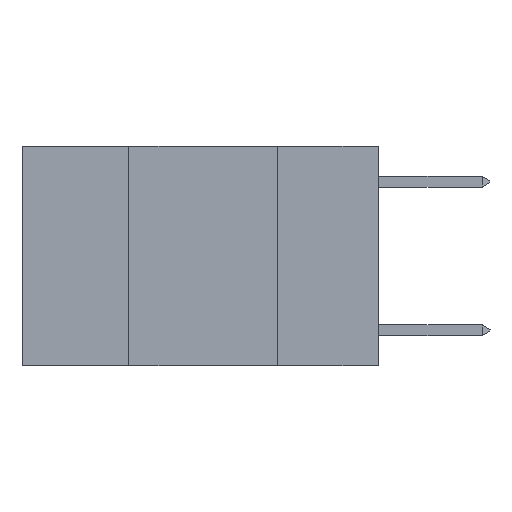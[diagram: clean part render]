
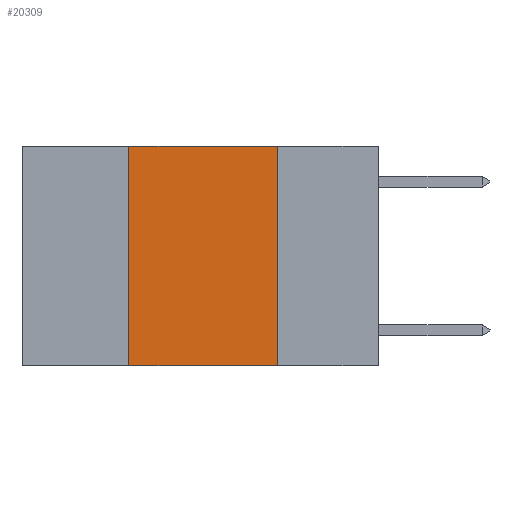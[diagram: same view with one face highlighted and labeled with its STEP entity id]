
A CAD part, left-side view. The second image highlights one B-rep face of the part: STEP entity #20309.
In plain terms, the highlighted planar face has unit normal (-1, 0, 0).
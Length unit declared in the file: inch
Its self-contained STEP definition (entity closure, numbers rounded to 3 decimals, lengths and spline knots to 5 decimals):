
#771 = FACE_OUTER_BOUND ( 'NONE', #905, .T. ) ;
#905 = EDGE_LOOP ( 'NONE', ( #24636, #25011, #25122, #25426 ) ) ;
#1793 = VERTEX_POINT ( 'NONE', #17961 ) ;
#1866 = LINE ( 'NONE', #19804, #6987 ) ;
#3017 = VECTOR ( 'NONE', #24069, 39.37008 ) ;
#3145 = PLANE ( 'NONE',  #8090 ) ;
#3482 = LINE ( 'NONE', #11906, #3017 ) ;
#3596 = CARTESIAN_POINT ( 'NONE',  ( 0., 0.42, 0. ) ) ;
#5006 = VERTEX_POINT ( 'NONE', #20461 ) ;
#6984 = CARTESIAN_POINT ( 'NONE',  ( 0., 0.42, 0. ) ) ;
#6987 = VECTOR ( 'NONE', #21824, 39.37008 ) ;
#8090 = AXIS2_PLACEMENT_3D ( 'NONE', #21835, #9604, #23850 ) ;
#8488 = LINE ( 'NONE', #6984, #24135 ) ;
#9604 = DIRECTION ( 'NONE',  ( 1., 0., 0. ) ) ;
#10487 = EDGE_CURVE ( 'NONE', #14197, #1793, #3482, .T. ) ;
#10814 = CARTESIAN_POINT ( 'NONE',  ( 0., 0.17, -0.37 ) ) ;
#11906 = CARTESIAN_POINT ( 'NONE',  ( 0., 0.6, 0. ) ) ;
#14197 = VERTEX_POINT ( 'NONE', #3596 ) ;
#15179 = EDGE_CURVE ( 'NONE', #1793, #25349, #24142, .T. ) ;
#15314 = DIRECTION ( 'NONE',  ( 0., 0., 1. ) ) ;
#17961 = CARTESIAN_POINT ( 'NONE',  ( 0., 0.17, 0. ) ) ;
#19154 = EDGE_CURVE ( 'NONE', #5006, #25349, #1866, .T. ) ;
#19804 = CARTESIAN_POINT ( 'NONE',  ( 0., 0.6, -0.37 ) ) ;
#20309 = ADVANCED_FACE ( 'NONE', ( #771 ), #3145, .F. ) ;
#20461 = CARTESIAN_POINT ( 'NONE',  ( 0., 0.42, -0.37 ) ) ;
#21824 = DIRECTION ( 'NONE',  ( 0., -1., 0. ) ) ;
#21835 = CARTESIAN_POINT ( 'NONE',  ( 0., 0.6, 0. ) ) ;
#21964 = CARTESIAN_POINT ( 'NONE',  ( 0., 0.17, 0. ) ) ;
#22845 = VECTOR ( 'NONE', #24003, 39.37008 ) ;
#23850 = DIRECTION ( 'NONE',  ( 0., 0., -1. ) ) ;
#24003 = DIRECTION ( 'NONE',  ( 0., 0., -1. ) ) ;
#24069 = DIRECTION ( 'NONE',  ( 0., -1., 0. ) ) ;
#24135 = VECTOR ( 'NONE', #15314, 39.37008 ) ;
#24142 = LINE ( 'NONE', #21964, #22845 ) ;
#24636 = ORIENTED_EDGE ( 'NONE', *, *, #15179, .F. ) ;
#24855 = EDGE_CURVE ( 'NONE', #5006, #14197, #8488, .T. ) ;
#25011 = ORIENTED_EDGE ( 'NONE', *, *, #10487, .F. ) ;
#25122 = ORIENTED_EDGE ( 'NONE', *, *, #24855, .F. ) ;
#25349 = VERTEX_POINT ( 'NONE', #10814 ) ;
#25426 = ORIENTED_EDGE ( 'NONE', *, *, #19154, .T. ) ;
